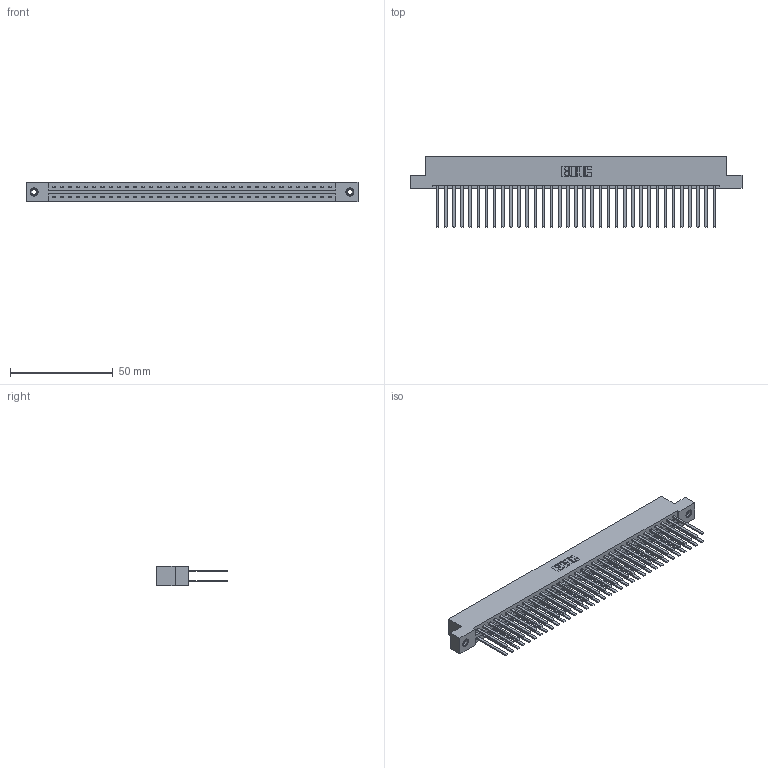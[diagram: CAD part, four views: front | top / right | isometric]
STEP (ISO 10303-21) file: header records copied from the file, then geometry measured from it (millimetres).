
FILE_DESCRIPTION (( 'STEP AP203' ), '1' );
FILE_NAME ('387-070-544-208.STEP', '2019-10-21T22:44:09', ( '' ), ( '' ), 'SwSTEP 2.0', 'SolidWorks 2016', '' );
FILE_SCHEMA (( 'CONFIG_CONTROL_DESIGN' ));
Length unit declared in the file: inch
Products named in the file (4): 345-292-001_345-293-144; 387-070-544-208; 345-250-001_345-250-003-102; 337 Part_Flush Mounting Lugs - 0.156 Dia-TI
Assembly tree (73 placements, depth 2):
  387-070-544-208
    337 Part_Flush Mounting Lugs - 0.156 Dia-TI
    345-292-001_345-293-144  x70
    345-250-001_345-250-003-102  x2
Bounding box: 161.7 x 34.3 x 9.4 mm (x, y, z)
Volume: 17922.4 mm3; surface area: 23422.8 mm2
Topology: 73 solids, 73 shells, 3534 faces, 10457 edges, 6870 vertices
Faces by surface type: plane 2482, cylinder 1036, cone 12, torus 4
Entity records: 29044 total; most frequent: CARTESIAN_POINT 4877, ORIENTED_EDGE 4806, DIRECTION 4189, EDGE_CURVE 2403, VECTOR 2259, LINE 2259, VERTEX_POINT 1596, AXIS2_PLACEMENT_3D 965
